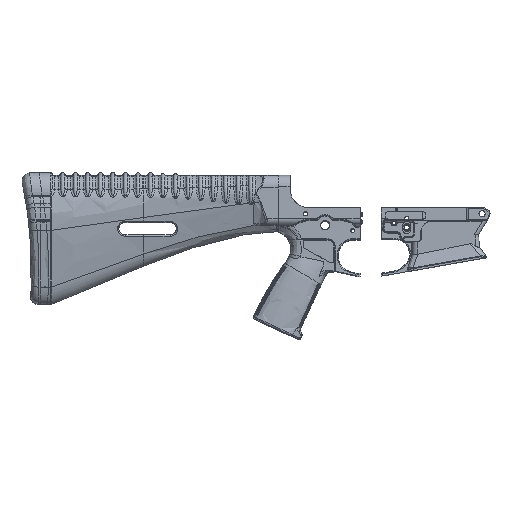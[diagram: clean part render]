
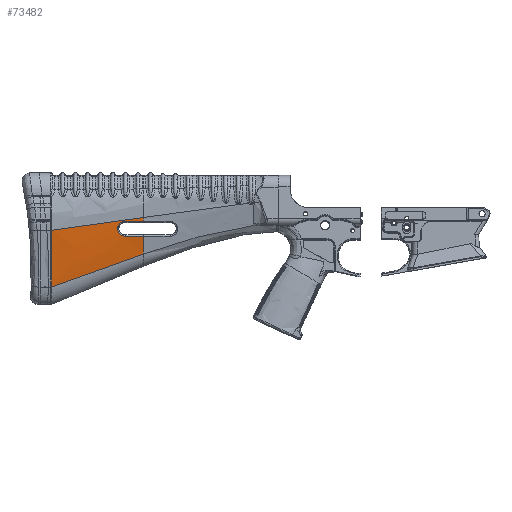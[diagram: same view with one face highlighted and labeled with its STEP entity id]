
A CAD part, top view. The second image highlights one B-rep face of the part: STEP entity #73482.
In plain terms, the highlighted free-form (B-spline) face has degree [3, 3] with [4, 4] control points.
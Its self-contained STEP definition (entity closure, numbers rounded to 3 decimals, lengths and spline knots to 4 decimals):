
#948=B_SPLINE_SURFACE_WITH_KNOTS('',3,3,((#121778,#121779,#121780,#121781),
(#121782,#121783,#121784,#121785),(#121786,#121787,#121788,#121789),(#121790,
#121791,#121792,#121793)),.UNSPECIFIED.,.F.,.F.,.F.,(4,4),(4,4),(0.,1.),
(0.4776,0.9165),.UNSPECIFIED.);
#2722=B_SPLINE_CURVE_WITH_KNOTS('',3,(#117870,#117871,#117872,#117873),
 .UNSPECIFIED.,.F.,.F.,(4,4),(-4.7135,-2.8128),
 .UNSPECIFIED.);
#2724=B_SPLINE_CURVE_WITH_KNOTS('',3,(#117974,#117975,#117976,#117977),
 .UNSPECIFIED.,.F.,.F.,(4,4),(0.4776,0.9165),
 .UNSPECIFIED.);
#2726=B_SPLINE_CURVE_WITH_KNOTS('',3,(#117995,#117996,#117997,#117998,#117999,
#118000),.UNSPECIFIED.,.F.,.F.,(4,2,4),(-5.9816,-3.0156,
0.),.UNSPECIFIED.);
#2819=B_SPLINE_CURVE_WITH_KNOTS('',3,(#121300,#121301,#121302,#121303),
 .UNSPECIFIED.,.F.,.F.,(4,4),(-3.8838,-1.9694),
 .UNSPECIFIED.);
#2828=B_SPLINE_CURVE_WITH_KNOTS('',3,(#121673,#121674,#121675,#121676,#121677,
#121678,#121679,#121680,#121681,#121682),.UNSPECIFIED.,.F.,.F.,(4,1,1,1,
1,1,1,4),(-2.4106,-2.0663,-1.7219,-1.3775,
-1.0331,-0.6888,-0.3444,0.),
 .UNSPECIFIED.);
#2830=B_SPLINE_CURVE_WITH_KNOTS('',3,(#121796,#121797,#121798,#121799),
 .UNSPECIFIED.,.F.,.F.,(4,4),(-0.4164,0.),.UNSPECIFIED.);
#2831=B_SPLINE_CURVE_WITH_KNOTS('',3,(#121800,#121801,#121802,#121803),
 .UNSPECIFIED.,.F.,.F.,(4,4),(0.4807,0.9156),
 .UNSPECIFIED.);
#2832=B_SPLINE_CURVE_WITH_KNOTS('',3,(#121804,#121805,#121806,#121807),
 .UNSPECIFIED.,.F.,.F.,(4,4),(-1.9008,0.),.UNSPECIFIED.);
#12067=FACE_OUTER_BOUND('',#16417,.T.);
#16417=EDGE_LOOP('',(#51532,#51533,#51534,#51535,#51536,#51537,#51538,#51539));
#28596=VERTEX_POINT('',#115158);
#28768=VERTEX_POINT('',#117836);
#28769=VERTEX_POINT('',#117868);
#28771=VERTEX_POINT('',#117963);
#28772=VERTEX_POINT('',#117994);
#28836=VERTEX_POINT('',#121671);
#28841=VERTEX_POINT('',#121794);
#28842=VERTEX_POINT('',#121795);
#37322=EDGE_CURVE('',#28769,#28768,#2722,.T.);
#37324=EDGE_CURVE('',#28771,#28596,#2724,.T.);
#37326=EDGE_CURVE('',#28772,#28596,#2726,.F.);
#37427=EDGE_CURVE('',#28771,#28768,#2819,.T.);
#37442=EDGE_CURVE('',#28836,#28769,#2828,.T.);
#37455=EDGE_CURVE('',#28841,#28842,#2830,.T.);
#37456=EDGE_CURVE('',#28842,#28772,#2831,.T.);
#37457=EDGE_CURVE('',#28841,#28836,#2832,.T.);
#51532=ORIENTED_EDGE('',*,*,#37455,.T.);
#51533=ORIENTED_EDGE('',*,*,#37456,.T.);
#51534=ORIENTED_EDGE('',*,*,#37326,.T.);
#51535=ORIENTED_EDGE('',*,*,#37324,.F.);
#51536=ORIENTED_EDGE('',*,*,#37427,.T.);
#51537=ORIENTED_EDGE('',*,*,#37322,.F.);
#51538=ORIENTED_EDGE('',*,*,#37442,.F.);
#51539=ORIENTED_EDGE('',*,*,#37457,.F.);
#73482=ADVANCED_FACE('',(#12067),#948,.F.);
#115158=CARTESIAN_POINT('',(-18.0335,-3.0038,-11.3765));
#117836=CARTESIAN_POINT('',(-14.2642,-0.9191,-11.2697));
#117868=CARTESIAN_POINT('',(-15.0107,-0.918,-11.2142));
#117870=CARTESIAN_POINT('Ctrl Pts',(-15.0107,-0.918,
-11.2142));
#117871=CARTESIAN_POINT('Ctrl Pts',(-14.7618,-0.9183,
-11.2321));
#117872=CARTESIAN_POINT('Ctrl Pts',(-14.513,-0.9187,
-11.2505));
#117873=CARTESIAN_POINT('Ctrl Pts',(-14.2642,-0.9191,
-11.2697));
#117963=CARTESIAN_POINT('',(-14.2642,-1.6534,-11.4406));
#117974=CARTESIAN_POINT('Ctrl Pts',(-14.2642,-1.6534,
-11.4406));
#117975=CARTESIAN_POINT('Ctrl Pts',(-15.9171,-2.229,
-11.4133));
#117976=CARTESIAN_POINT('Ctrl Pts',(-17.3565,-2.8272,
-11.3849));
#117977=CARTESIAN_POINT('Ctrl Pts',(-18.0335,-3.0038,
-11.3765));
#117994=CARTESIAN_POINT('',(-18.0335,-0.6789,-11.0043));
#117995=CARTESIAN_POINT('Ctrl Pts',(-18.0335,-3.0038,
-11.3765));
#117996=CARTESIAN_POINT('Ctrl Pts',(-18.0335,-2.6238,
-11.2926));
#117997=CARTESIAN_POINT('Ctrl Pts',(-18.0335,-2.2407,
-11.2201));
#117998=CARTESIAN_POINT('Ctrl Pts',(-18.0335,-1.4656,
-11.096));
#117999=CARTESIAN_POINT('Ctrl Pts',(-18.0335,-1.0726,
-11.0447));
#118000=CARTESIAN_POINT('Ctrl Pts',(-18.0335,-0.6789,
-11.0043));
#121300=CARTESIAN_POINT('Ctrl Pts',(-14.2642,-1.6534,
-11.4406));
#121301=CARTESIAN_POINT('Ctrl Pts',(-14.2642,-1.4106,
-11.3763));
#121302=CARTESIAN_POINT('Ctrl Pts',(-14.2642,-1.1654,
-11.3193));
#121303=CARTESIAN_POINT('Ctrl Pts',(-14.2642,-0.9191,
-11.2697));
#121671=CARTESIAN_POINT('',(-15.0115,-0.3159,-11.1207));
#121673=CARTESIAN_POINT('Ctrl Pts',(-15.0115,-0.3159,
-11.1207));
#121674=CARTESIAN_POINT('Ctrl Pts',(-15.0566,-0.3159,
-11.1182));
#121675=CARTESIAN_POINT('Ctrl Pts',(-15.147,-0.3366,
-11.116));
#121676=CARTESIAN_POINT('Ctrl Pts',(-15.2553,-0.424,
-11.1216));
#121677=CARTESIAN_POINT('Ctrl Pts',(-15.3142,-0.5494,
-11.1355));
#121678=CARTESIAN_POINT('Ctrl Pts',(-15.3131,-0.6874,
-11.1558));
#121679=CARTESIAN_POINT('Ctrl Pts',(-15.2531,-0.811,
-11.1792));
#121680=CARTESIAN_POINT('Ctrl Pts',(-15.1457,-0.897,
-11.2009));
#121681=CARTESIAN_POINT('Ctrl Pts',(-15.0558,-0.9179,
-11.211));
#121682=CARTESIAN_POINT('Ctrl Pts',(-15.0107,-0.918,
-11.2142));
#121778=CARTESIAN_POINT('Ctrl Pts',(-14.2289,-0.1498,
-11.1402));
#121779=CARTESIAN_POINT('Ctrl Pts',(-15.897,-0.3806,
-11.0847));
#121780=CARTESIAN_POINT('Ctrl Pts',(-17.3619,-0.5864,
-11.0201));
#121781=CARTESIAN_POINT('Ctrl Pts',(-18.0375,-0.6795,
-11.0042));
#121782=CARTESIAN_POINT('Ctrl Pts',(-14.2407,-0.6622,
-11.2121));
#121783=CARTESIAN_POINT('Ctrl Pts',(-15.9037,-1.0102,
-11.1606));
#121784=CARTESIAN_POINT('Ctrl Pts',(-17.3601,-1.3495,
-11.1));
#121785=CARTESIAN_POINT('Ctrl Pts',(-18.0362,-1.4721,
-11.0855));
#121786=CARTESIAN_POINT('Ctrl Pts',(-14.2524,-1.1649,
-11.3124));
#121787=CARTESIAN_POINT('Ctrl Pts',(-15.9104,-1.6288,
-11.2703));
#121788=CARTESIAN_POINT('Ctrl Pts',(-17.3583,-2.1006,
-11.222));
#121789=CARTESIAN_POINT('Ctrl Pts',(-18.0348,-2.2516,
-11.2103));
#121790=CARTESIAN_POINT('Ctrl Pts',(-14.2642,-1.6534,
-11.4406));
#121791=CARTESIAN_POINT('Ctrl Pts',(-15.9171,-2.229,
-11.4133));
#121792=CARTESIAN_POINT('Ctrl Pts',(-17.3565,-2.8272,
-11.3849));
#121793=CARTESIAN_POINT('Ctrl Pts',(-18.0335,-3.0038,
-11.3765));
#121794=CARTESIAN_POINT('',(-14.2642,-0.3169,-11.1629));
#121795=CARTESIAN_POINT('',(-14.2642,-0.1546,-11.139));
#121796=CARTESIAN_POINT('Ctrl Pts',(-14.2642,-0.3169,
-11.1629));
#121797=CARTESIAN_POINT('Ctrl Pts',(-14.2642,-0.2628,
-11.1546));
#121798=CARTESIAN_POINT('Ctrl Pts',(-14.2642,-0.2088,
-11.1466));
#121799=CARTESIAN_POINT('Ctrl Pts',(-14.2642,-0.1546,
-11.139));
#121800=CARTESIAN_POINT('Ctrl Pts',(-14.2642,-0.1546,
-11.139));
#121801=CARTESIAN_POINT('Ctrl Pts',(-15.9143,-0.3831,
-11.0839));
#121802=CARTESIAN_POINT('Ctrl Pts',(-17.3609,-0.5862,
-11.0202));
#121803=CARTESIAN_POINT('Ctrl Pts',(-18.0335,-0.6789,
-11.0043));
#121804=CARTESIAN_POINT('Ctrl Pts',(-14.2642,-0.3169,
-11.1629));
#121805=CARTESIAN_POINT('Ctrl Pts',(-14.5133,-0.3165,
-11.1486));
#121806=CARTESIAN_POINT('Ctrl Pts',(-14.7624,-0.3162,
-11.1345));
#121807=CARTESIAN_POINT('Ctrl Pts',(-15.0115,-0.3159,
-11.1207));
